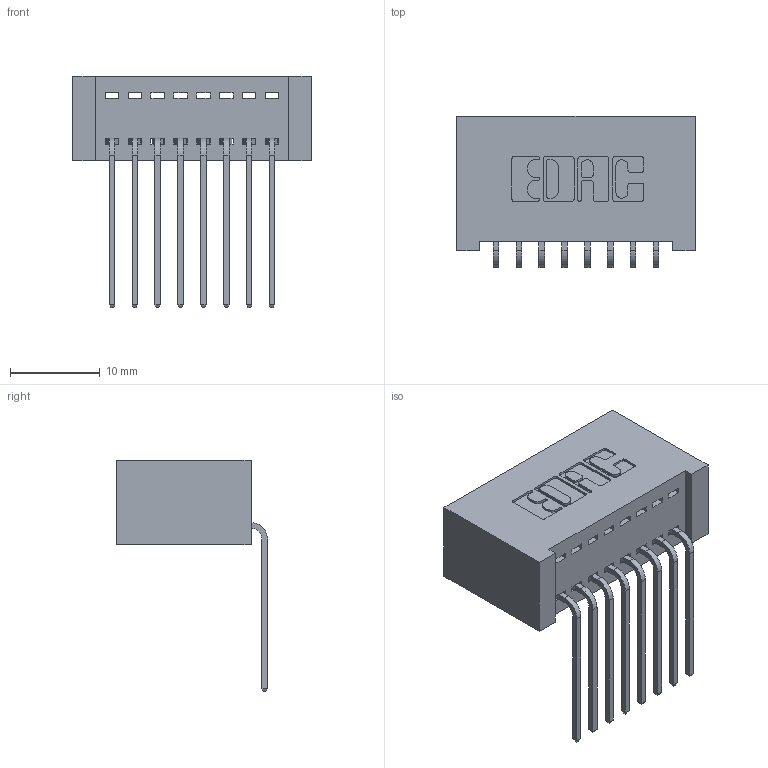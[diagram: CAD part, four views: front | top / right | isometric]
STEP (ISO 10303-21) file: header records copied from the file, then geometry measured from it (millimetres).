
FILE_DESCRIPTION (( 'STEP AP203' ), '1' );
FILE_NAME ('392-008-559-101.STEP', '2019-10-05T00:02:56', ( '' ), ( '' ), 'SwSTEP 2.0', 'SolidWorks 2016', '' );
FILE_SCHEMA (( 'CONFIG_CONTROL_DESIGN' ));
Length unit declared in the file: inch
Products named in the file (3): 342 Part_Lugless; 345-292-001_558 559 Tail - 1; 392-008-559-101
Assembly tree (9 placements, depth 2):
  392-008-559-101
    342 Part_Lugless
    345-292-001_558 559 Tail - 1  x8
Bounding box: 26.57 x 16.83 x 25.78 mm (x, y, z)
Volume: 2639.9 mm3; surface area: 3716.4 mm2
Topology: 9 solids, 9 shells, 582 faces, 1731 edges, 1142 vertices
Faces by surface type: plane 414, cylinder 168
Entity records: 8963 total; most frequent: CARTESIAN_POINT 1558, ORIENTED_EDGE 1502, DIRECTION 1375, EDGE_CURVE 751, VECTOR 631, LINE 631, VERTEX_POINT 498, AXIS2_PLACEMENT_3D 372
